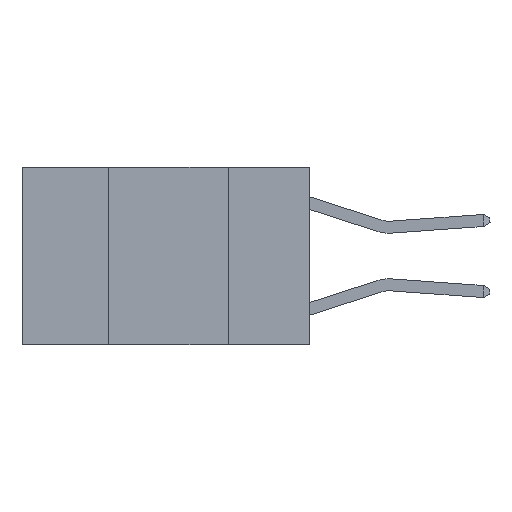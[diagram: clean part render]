
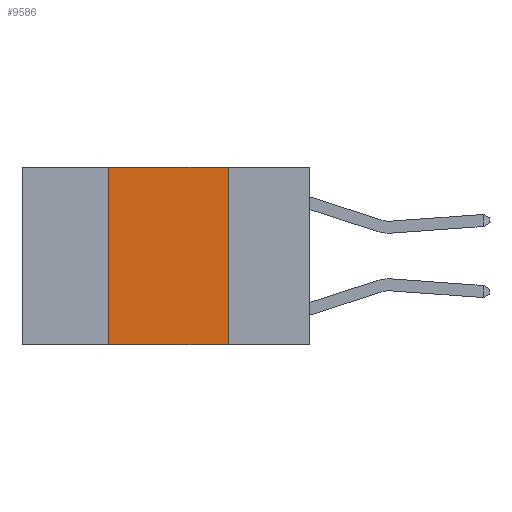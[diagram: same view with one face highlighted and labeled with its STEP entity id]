
A CAD part, left-side view. The second image highlights one B-rep face of the part: STEP entity #9586.
In plain terms, the highlighted planar face has unit normal (-1, 0, 0).
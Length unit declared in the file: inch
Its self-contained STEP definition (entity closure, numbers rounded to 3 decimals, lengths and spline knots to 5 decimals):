
#12 = DIRECTION ( 'NONE',  ( 0., 0., -1. ) ) ;
#444 = EDGE_CURVE ( 'NONE', #939, #10258, #2485, .T. ) ;
#456 = VECTOR ( 'NONE', #7534, 39.37008 ) ;
#939 = VERTEX_POINT ( 'NONE', #7074 ) ;
#1644 = CARTESIAN_POINT ( 'NONE',  ( 0., 0.6, 0. ) ) ;
#1892 = FACE_OUTER_BOUND ( 'NONE', #9620, .T. ) ;
#1933 = LINE ( 'NONE', #6431, #6139 ) ;
#2212 = EDGE_CURVE ( 'NONE', #5188, #8540, #1933, .T. ) ;
#2220 = LINE ( 'NONE', #5834, #4100 ) ;
#2252 = CARTESIAN_POINT ( 'NONE',  ( 0., 0.6, -0.37 ) ) ;
#2278 = ORIENTED_EDGE ( 'NONE', *, *, #444, .F. ) ;
#2485 = LINE ( 'NONE', #6052, #8669 ) ;
#2539 = ORIENTED_EDGE ( 'NONE', *, *, #2212, .F. ) ;
#2640 = LINE ( 'NONE', #2252, #456 ) ;
#3255 = PLANE ( 'NONE',  #10394 ) ;
#3358 = DIRECTION ( 'NONE',  ( 0., 0., 1. ) ) ;
#4100 = VECTOR ( 'NONE', #7733, 39.37008 ) ;
#4124 = CARTESIAN_POINT ( 'NONE',  ( 0., 0.17, -0.37 ) ) ;
#4642 = EDGE_CURVE ( 'NONE', #5188, #10258, #2640, .T. ) ;
#4864 = DIRECTION ( 'NONE',  ( 1., 0., 0. ) ) ;
#5188 = VERTEX_POINT ( 'NONE', #5384 ) ;
#5384 = CARTESIAN_POINT ( 'NONE',  ( 0., 0.42, -0.37 ) ) ;
#5834 = CARTESIAN_POINT ( 'NONE',  ( 0., 0.6, 0. ) ) ;
#6052 = CARTESIAN_POINT ( 'NONE',  ( 0., 0.17, 0. ) ) ;
#6139 = VECTOR ( 'NONE', #3358, 39.37008 ) ;
#6431 = CARTESIAN_POINT ( 'NONE',  ( 0., 0.42, 0. ) ) ;
#6484 = ORIENTED_EDGE ( 'NONE', *, *, #6856, .F. ) ;
#6719 = ORIENTED_EDGE ( 'NONE', *, *, #4642, .T. ) ;
#6856 = EDGE_CURVE ( 'NONE', #8540, #939, #2220, .T. ) ;
#7074 = CARTESIAN_POINT ( 'NONE',  ( 0., 0.17, 0. ) ) ;
#7525 = CARTESIAN_POINT ( 'NONE',  ( 0., 0.42, 0. ) ) ;
#7534 = DIRECTION ( 'NONE',  ( 0., -1., 0. ) ) ;
#7733 = DIRECTION ( 'NONE',  ( 0., -1., 0. ) ) ;
#8540 = VERTEX_POINT ( 'NONE', #7525 ) ;
#8669 = VECTOR ( 'NONE', #10454, 39.37008 ) ;
#9586 = ADVANCED_FACE ( 'NONE', ( #1892 ), #3255, .F. ) ;
#9620 = EDGE_LOOP ( 'NONE', ( #2278, #6484, #2539, #6719 ) ) ;
#10258 = VERTEX_POINT ( 'NONE', #4124 ) ;
#10394 = AXIS2_PLACEMENT_3D ( 'NONE', #1644, #4864, #12 ) ;
#10454 = DIRECTION ( 'NONE',  ( 0., 0., -1. ) ) ;
